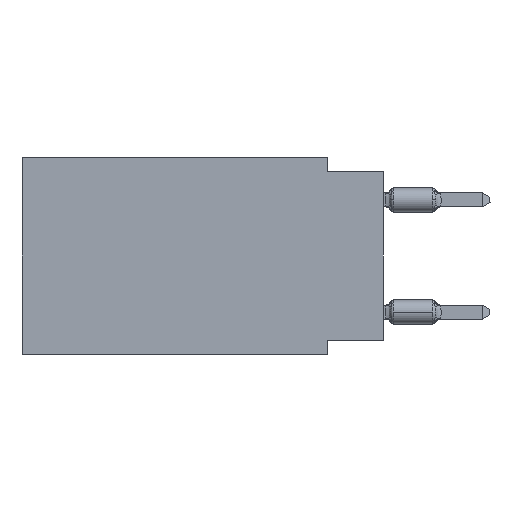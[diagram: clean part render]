
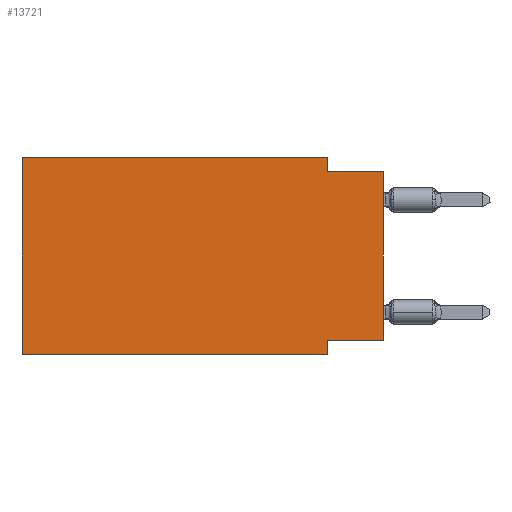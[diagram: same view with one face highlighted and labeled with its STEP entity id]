
A CAD part, left-side view. The second image highlights one B-rep face of the part: STEP entity #13721.
In plain terms, the highlighted planar face has unit normal (-1, 0, 0).
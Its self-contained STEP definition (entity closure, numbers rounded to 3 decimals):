
#124 = VECTOR ( 'NONE', #31790, 1000. ) ;
#211 = VERTEX_POINT ( 'NONE', #29275 ) ;
#1294 = CARTESIAN_POINT ( 'NONE',  ( 0., 16.383, 0. ) ) ;
#1569 = EDGE_CURVE ( 'NONE', #13430, #7715, #15392, .T. ) ;
#1626 = FACE_OUTER_BOUND ( 'NONE', #16858, .T. ) ;
#1653 = CARTESIAN_POINT ( 'NONE',  ( 0., 16.383, -8.89 ) ) ;
#1654 = AXIS2_PLACEMENT_3D ( 'NONE', #1954, #4251, #27339 ) ;
#1954 = CARTESIAN_POINT ( 'NONE',  ( 0., 16.383, 0. ) ) ;
#2008 = ORIENTED_EDGE ( 'NONE', *, *, #1569, .T. ) ;
#2522 = DIRECTION ( 'NONE',  ( 0., 0., -1. ) ) ;
#3860 = DIRECTION ( 'NONE',  ( 0., -1., 0. ) ) ;
#3920 = LINE ( 'NONE', #1294, #18799 ) ;
#4123 = VERTEX_POINT ( 'NONE', #5497 ) ;
#4251 = DIRECTION ( 'NONE',  ( 1., 0., 0. ) ) ;
#4640 = LINE ( 'NONE', #19460, #19079 ) ;
#5497 = CARTESIAN_POINT ( 'NONE',  ( 0., 2.54, -8.255 ) ) ;
#5579 = LINE ( 'NONE', #15456, #25795 ) ;
#6706 = EDGE_CURVE ( 'NONE', #211, #14523, #4640, .T. ) ;
#6760 = CARTESIAN_POINT ( 'NONE',  ( 0., 16.383, -8.89 ) ) ;
#6771 = ORIENTED_EDGE ( 'NONE', *, *, #11496, .F. ) ;
#7715 = VERTEX_POINT ( 'NONE', #12701 ) ;
#9827 = CARTESIAN_POINT ( 'NONE',  ( 0., 0., 0. ) ) ;
#10342 = DIRECTION ( 'NONE',  ( 0., 0., -1. ) ) ;
#10379 = VECTOR ( 'NONE', #10342, 1000. ) ;
#11110 = DIRECTION ( 'NONE',  ( 0., 0., 1. ) ) ;
#11496 = EDGE_CURVE ( 'NONE', #4123, #31794, #15109, .T. ) ;
#12015 = PLANE ( 'NONE',  #1654 ) ;
#12208 = ORIENTED_EDGE ( 'NONE', *, *, #12327, .F. ) ;
#12327 = EDGE_CURVE ( 'NONE', #21758, #211, #3920, .T. ) ;
#12701 = CARTESIAN_POINT ( 'NONE',  ( 0., 0., -0.635 ) ) ;
#13427 = EDGE_CURVE ( 'NONE', #14523, #30881, #27104, .T. ) ;
#13430 = VERTEX_POINT ( 'NONE', #22781 ) ;
#13721 = ADVANCED_FACE ( 'NONE', ( #1626 ), #12015, .F. ) ;
#13983 = VECTOR ( 'NONE', #11110, 1000. ) ;
#14273 = VECTOR ( 'NONE', #2522, 1000. ) ;
#14523 = VERTEX_POINT ( 'NONE', #28277 ) ;
#15109 = LINE ( 'NONE', #22372, #10379 ) ;
#15392 = LINE ( 'NONE', #9827, #13983 ) ;
#15456 = CARTESIAN_POINT ( 'NONE',  ( 0., 0., -8.255 ) ) ;
#16486 = ORIENTED_EDGE ( 'NONE', *, *, #6706, .F. ) ;
#16631 = VECTOR ( 'NONE', #3860, 1000. ) ;
#16858 = EDGE_LOOP ( 'NONE', ( #2008, #24866, #17509, #16486, #12208, #21551, #6771, #29670 ) ) ;
#17509 = ORIENTED_EDGE ( 'NONE', *, *, #13427, .F. ) ;
#18240 = CARTESIAN_POINT ( 'NONE',  ( 0., 2.54, -8.89 ) ) ;
#18417 = DIRECTION ( 'NONE',  ( 0., 0., 1. ) ) ;
#18436 = EDGE_CURVE ( 'NONE', #13430, #4123, #5579, .T. ) ;
#18799 = VECTOR ( 'NONE', #18417, 1000. ) ;
#18851 = CARTESIAN_POINT ( 'NONE',  ( 0., 0., -0.635 ) ) ;
#19079 = VECTOR ( 'NONE', #29526, 1000. ) ;
#19460 = CARTESIAN_POINT ( 'NONE',  ( 0., 16.383, 0. ) ) ;
#20758 = EDGE_CURVE ( 'NONE', #30881, #7715, #25971, .T. ) ;
#21551 = ORIENTED_EDGE ( 'NONE', *, *, #26721, .T. ) ;
#21758 = VERTEX_POINT ( 'NONE', #6760 ) ;
#22372 = CARTESIAN_POINT ( 'NONE',  ( 0., 2.54, -8.89 ) ) ;
#22781 = CARTESIAN_POINT ( 'NONE',  ( 0., 0., -8.255 ) ) ;
#24239 = LINE ( 'NONE', #1653, #124 ) ;
#24866 = ORIENTED_EDGE ( 'NONE', *, *, #20758, .F. ) ;
#25648 = CARTESIAN_POINT ( 'NONE',  ( 0., 2.54, -0.635 ) ) ;
#25704 = DIRECTION ( 'NONE',  ( 0., 1., 0. ) ) ;
#25795 = VECTOR ( 'NONE', #25704, 1000. ) ;
#25971 = LINE ( 'NONE', #18851, #16631 ) ;
#26721 = EDGE_CURVE ( 'NONE', #21758, #31794, #24239, .T. ) ;
#27104 = LINE ( 'NONE', #30362, #14273 ) ;
#27339 = DIRECTION ( 'NONE',  ( 0., 0., -1. ) ) ;
#28277 = CARTESIAN_POINT ( 'NONE',  ( 0., 2.54, 0. ) ) ;
#29275 = CARTESIAN_POINT ( 'NONE',  ( 0., 16.383, 0. ) ) ;
#29526 = DIRECTION ( 'NONE',  ( 0., -1., 0. ) ) ;
#29670 = ORIENTED_EDGE ( 'NONE', *, *, #18436, .F. ) ;
#30362 = CARTESIAN_POINT ( 'NONE',  ( 0., 2.54, 0. ) ) ;
#30881 = VERTEX_POINT ( 'NONE', #25648 ) ;
#31790 = DIRECTION ( 'NONE',  ( 0., -1., 0. ) ) ;
#31794 = VERTEX_POINT ( 'NONE', #18240 ) ;
